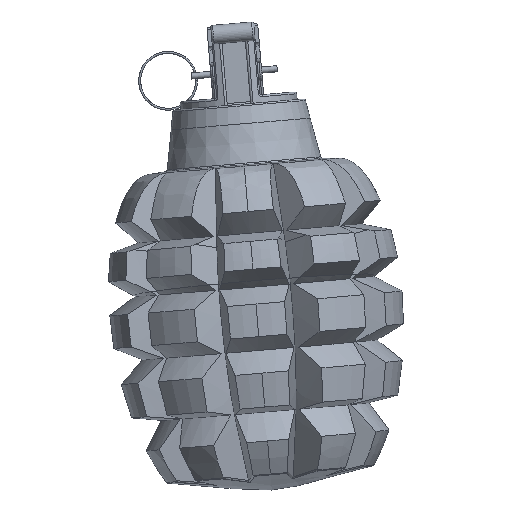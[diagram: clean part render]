
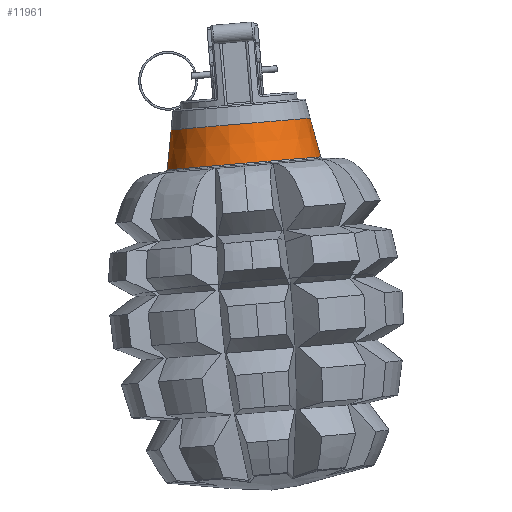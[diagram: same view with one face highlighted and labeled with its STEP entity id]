
A CAD part, top view. The second image highlights one B-rep face of the part: STEP entity #11961.
In plain terms, the highlighted conical face has half-angle 10.378 degrees and reference radius 16.964 mm.
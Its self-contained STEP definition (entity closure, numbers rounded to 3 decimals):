
#4064 = AXIS2_PLACEMENT_3D ( 'NONE', #6144, #6148, #6149 ) ;
#4071 = VECTOR ( 'NONE', #6147, 1000. ) ;
#4074 = VECTOR ( 'NONE', #6179, 1000. ) ;
#5392 = CARTESIAN_POINT ( 'NONE',  ( 111.407, 118.894, -0.004 ) ) ;
#5397 = CARTESIAN_POINT ( 'NONE',  ( 112.395, 129.12, -0.004 ) ) ;
#5440 = CARTESIAN_POINT ( 'NONE',  ( 148.031, 132.151, -0.004 ) ) ;
#5460 = CARTESIAN_POINT ( 'NONE',  ( 150.731, 122.239, -0.004 ) ) ;
#6144 = CARTESIAN_POINT ( 'NONE',  ( 131.069, 120.567, -0.004 ) ) ;
#6145 = LINE ( 'NONE', #6146, #4071 ) ;
#6146 = CARTESIAN_POINT ( 'NONE',  ( 112.885, 134.194, -0.004 ) ) ;
#6147 = DIRECTION ( 'NONE',  ( -0.096, -0.995, 0. ) ) ;
#6148 = DIRECTION ( 'NONE',  ( -0.085, 0.996, 0. ) ) ;
#6149 = DIRECTION ( 'NONE',  ( 0.996, 0.085, 0. ) ) ;
#6177 = LINE ( 'NONE', #6178, #4074 ) ;
#6178 = CARTESIAN_POINT ( 'NONE',  ( 146.691, 137.07, -0.004 ) ) ;
#6179 = DIRECTION ( 'NONE',  ( 0.263, -0.965, 0. ) ) ;
#9678 = ORIENTED_EDGE ( 'NONE', *, *, #17475, .T. ) ;
#9679 = ORIENTED_EDGE ( 'NONE', *, *, #17479, .F. ) ;
#9688 = ORIENTED_EDGE ( 'NONE', *, *, #11855, .T. ) ;
#9694 = ORIENTED_EDGE ( 'NONE', *, *, #17476, .T. ) ;
#11855 = EDGE_CURVE ( 'NONE', #14618, #14575, #13803, .T. ) ;
#11961 = ADVANCED_FACE ( 'NONE', ( #26064 ), #13846, .T. ) ;
#13803 = CIRCLE ( 'NONE', #25976, 17.882 ) ;
#13846 = CONICAL_SURFACE ( 'NONE', #26071, 16.964, 0.181 ) ;
#13935 = CIRCLE ( 'NONE', #4064, 19.733 ) ;
#14570 = VERTEX_POINT ( 'NONE', #5392 ) ;
#14575 = VERTEX_POINT ( 'NONE', #5397 ) ;
#14618 = VERTEX_POINT ( 'NONE', #5440 ) ;
#14638 = VERTEX_POINT ( 'NONE', #5460 ) ;
#14669 = EDGE_LOOP ( 'NONE', ( #9688, #9678, #9694, #9679 ) ) ;
#17475 = EDGE_CURVE ( 'NONE', #14575, #14570, #6145, .T. ) ;
#17476 = EDGE_CURVE ( 'NONE', #14570, #14638, #13935, .T. ) ;
#17479 = EDGE_CURVE ( 'NONE', #14618, #14638, #6177, .T. ) ;
#25171 = CARTESIAN_POINT ( 'NONE',  ( 130.213, 130.635, -0.004 ) ) ;
#25175 = DIRECTION ( 'NONE',  ( 0.085, -0.996, 0. ) ) ;
#25176 = DIRECTION ( 'NONE',  ( -0.996, -0.085, 0. ) ) ;
#25587 = CARTESIAN_POINT ( 'NONE',  ( 129.788, 135.632, -0.004 ) ) ;
#25588 = DIRECTION ( 'NONE',  ( 0.085, -0.996, 0. ) ) ;
#25589 = DIRECTION ( 'NONE',  ( 0.996, 0.085, 0. ) ) ;
#25976 = AXIS2_PLACEMENT_3D ( 'NONE', #25171, #25175, #25176 ) ;
#26064 = FACE_OUTER_BOUND ( 'NONE', #14669, .T. ) ;
#26071 = AXIS2_PLACEMENT_3D ( 'NONE', #25587, #25588, #25589 ) ;
